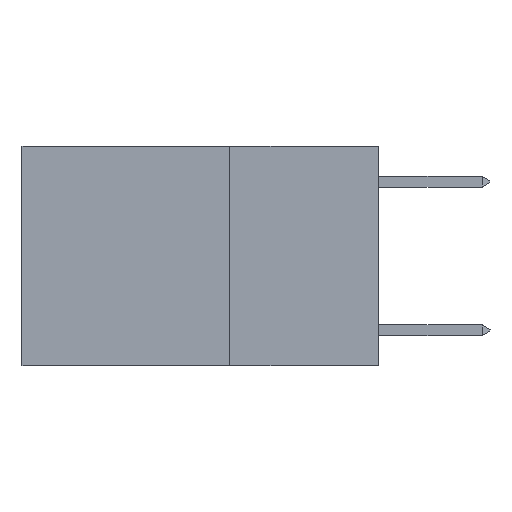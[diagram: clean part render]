
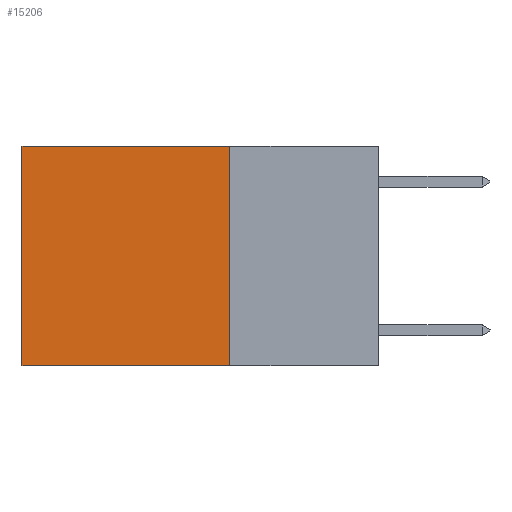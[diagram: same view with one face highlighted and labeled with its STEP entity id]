
A CAD part, left-side view. The second image highlights one B-rep face of the part: STEP entity #15206.
In plain terms, the highlighted planar face has unit normal (-1, 0, 0).
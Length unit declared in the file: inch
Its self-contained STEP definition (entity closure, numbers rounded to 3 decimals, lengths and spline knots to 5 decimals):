
#2027 = LINE ( 'NONE', #13187, #18098 ) ;
#2519 = EDGE_LOOP ( 'NONE', ( #4955, #11306, #13933, #16501 ) ) ;
#4729 = EDGE_CURVE ( 'NONE', #7835, #10336, #11775, .T. ) ;
#4955 = ORIENTED_EDGE ( 'NONE', *, *, #13554, .T. ) ;
#5376 = FACE_OUTER_BOUND ( 'NONE', #2519, .T. ) ;
#5861 = DIRECTION ( 'NONE',  ( 0., 1., 0. ) ) ;
#6146 = CARTESIAN_POINT ( 'NONE',  ( 0.2625, 0.25, 0. ) ) ;
#6458 = CARTESIAN_POINT ( 'NONE',  ( 0.2625, 0.25, 0. ) ) ;
#7610 = CARTESIAN_POINT ( 'NONE',  ( 0.2625, 0.6, -0.37 ) ) ;
#7835 = VERTEX_POINT ( 'NONE', #6458 ) ;
#9025 = VERTEX_POINT ( 'NONE', #17681 ) ;
#9189 = EDGE_CURVE ( 'NONE', #10336, #17697, #2027, .T. ) ;
#10336 = VERTEX_POINT ( 'NONE', #17636 ) ;
#10755 = DIRECTION ( 'NONE',  ( 0., 0., -1. ) ) ;
#10780 = DIRECTION ( 'NONE',  ( 1., 0., 0. ) ) ;
#10975 = PLANE ( 'NONE',  #18679 ) ;
#10993 = EDGE_CURVE ( 'NONE', #7835, #9025, #11085, .T. ) ;
#11085 = LINE ( 'NONE', #6146, #11445 ) ;
#11306 = ORIENTED_EDGE ( 'NONE', *, *, #9189, .F. ) ;
#11337 = CARTESIAN_POINT ( 'NONE',  ( 0.2625, 0.25, 0. ) ) ;
#11445 = VECTOR ( 'NONE', #5861, 39.37008 ) ;
#11459 = VECTOR ( 'NONE', #13924, 39.37008 ) ;
#11775 = LINE ( 'NONE', #14129, #11459 ) ;
#13129 = DIRECTION ( 'NONE',  ( 0., 1., 0. ) ) ;
#13187 = CARTESIAN_POINT ( 'NONE',  ( 0.2625, 0.25, -0.37 ) ) ;
#13232 = DIRECTION ( 'NONE',  ( 0., 0., -1. ) ) ;
#13254 = CARTESIAN_POINT ( 'NONE',  ( 0.2625, 0.6, 0. ) ) ;
#13554 = EDGE_CURVE ( 'NONE', #9025, #17697, #15048, .T. ) ;
#13924 = DIRECTION ( 'NONE',  ( 0., 0., -1. ) ) ;
#13933 = ORIENTED_EDGE ( 'NONE', *, *, #4729, .F. ) ;
#14129 = CARTESIAN_POINT ( 'NONE',  ( 0.2625, 0.25, 0. ) ) ;
#14637 = VECTOR ( 'NONE', #13232, 39.37008 ) ;
#15048 = LINE ( 'NONE', #13254, #14637 ) ;
#15206 = ADVANCED_FACE ( 'NONE', ( #5376 ), #10975, .F. ) ;
#16501 = ORIENTED_EDGE ( 'NONE', *, *, #10993, .T. ) ;
#17636 = CARTESIAN_POINT ( 'NONE',  ( 0.2625, 0.25, -0.37 ) ) ;
#17681 = CARTESIAN_POINT ( 'NONE',  ( 0.2625, 0.6, 0. ) ) ;
#17697 = VERTEX_POINT ( 'NONE', #7610 ) ;
#18098 = VECTOR ( 'NONE', #13129, 39.37008 ) ;
#18679 = AXIS2_PLACEMENT_3D ( 'NONE', #11337, #10780, #10755 ) ;
